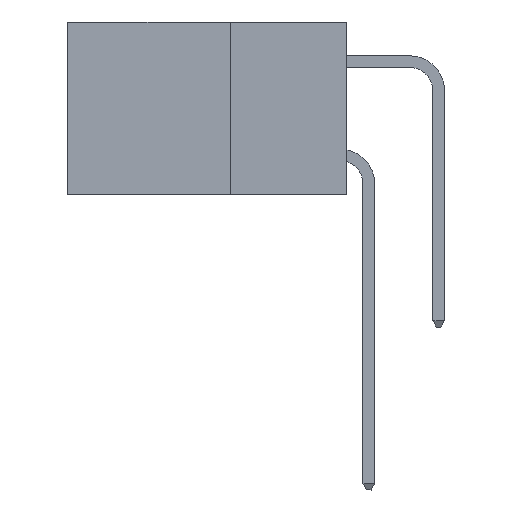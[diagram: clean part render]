
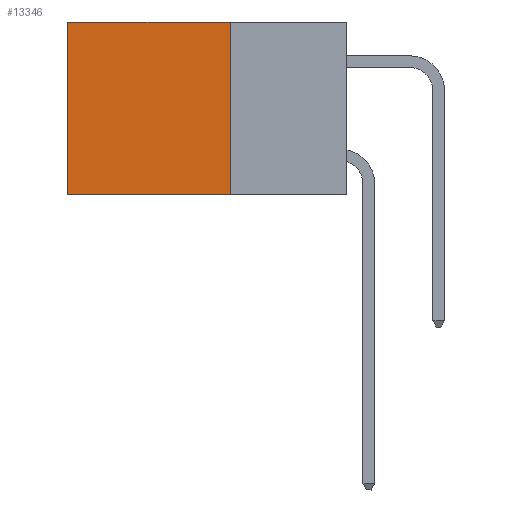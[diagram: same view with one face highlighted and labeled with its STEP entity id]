
A CAD part, left-side view. The second image highlights one B-rep face of the part: STEP entity #13346.
In plain terms, the highlighted planar face has unit normal (-1, 0, 0).
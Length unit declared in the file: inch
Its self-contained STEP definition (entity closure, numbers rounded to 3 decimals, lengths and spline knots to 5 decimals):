
#24 = LINE ( 'NONE', #17422, #7165 ) ;
#796 = DIRECTION ( 'NONE',  ( 0., 1., 0. ) ) ;
#1942 = DIRECTION ( 'NONE',  ( 0., 1., 0. ) ) ;
#2718 = LINE ( 'NONE', #18324, #11036 ) ;
#2976 = DIRECTION ( 'NONE',  ( 0., 0., -1. ) ) ;
#3465 = VECTOR ( 'NONE', #2976, 39.37008 ) ;
#4637 = CARTESIAN_POINT ( 'NONE',  ( 0.2875, 0.25, 0. ) ) ;
#5913 = AXIS2_PLACEMENT_3D ( 'NONE', #19322, #11659, #7561 ) ;
#7165 = VECTOR ( 'NONE', #1942, 39.37008 ) ;
#7546 = EDGE_CURVE ( 'NONE', #17994, #19937, #24, .T. ) ;
#7561 = DIRECTION ( 'NONE',  ( 0., 0., -1. ) ) ;
#7886 = CARTESIAN_POINT ( 'NONE',  ( 0.2875, 0.6, 0. ) ) ;
#10501 = CARTESIAN_POINT ( 'NONE',  ( 0.2875, 0.6, -0.37 ) ) ;
#11036 = VECTOR ( 'NONE', #796, 39.37008 ) ;
#11659 = DIRECTION ( 'NONE',  ( 1., 0., 0. ) ) ;
#12599 = EDGE_LOOP ( 'NONE', ( #22197, #15051, #13017, #24459 ) ) ;
#13017 = ORIENTED_EDGE ( 'NONE', *, *, #17005, .F. ) ;
#13346 = ADVANCED_FACE ( 'NONE', ( #22930 ), #25240, .F. ) ;
#14143 = LINE ( 'NONE', #7886, #21385 ) ;
#15051 = ORIENTED_EDGE ( 'NONE', *, *, #24342, .F. ) ;
#15618 = EDGE_CURVE ( 'NONE', #19937, #22128, #14143, .T. ) ;
#16440 = CARTESIAN_POINT ( 'NONE',  ( 0.2875, 0.25, 0. ) ) ;
#17005 = EDGE_CURVE ( 'NONE', #17994, #24749, #20509, .T. ) ;
#17422 = CARTESIAN_POINT ( 'NONE',  ( 0.2875, 0.25, 0. ) ) ;
#17994 = VERTEX_POINT ( 'NONE', #16440 ) ;
#18324 = CARTESIAN_POINT ( 'NONE',  ( 0.2875, 0.25, -0.37 ) ) ;
#19322 = CARTESIAN_POINT ( 'NONE',  ( 0.2875, 0.25, 0. ) ) ;
#19937 = VERTEX_POINT ( 'NONE', #24118 ) ;
#20509 = LINE ( 'NONE', #4637, #3465 ) ;
#20952 = CARTESIAN_POINT ( 'NONE',  ( 0.2875, 0.25, -0.37 ) ) ;
#21385 = VECTOR ( 'NONE', #21704, 39.37008 ) ;
#21704 = DIRECTION ( 'NONE',  ( 0., 0., -1. ) ) ;
#22128 = VERTEX_POINT ( 'NONE', #10501 ) ;
#22197 = ORIENTED_EDGE ( 'NONE', *, *, #15618, .T. ) ;
#22930 = FACE_OUTER_BOUND ( 'NONE', #12599, .T. ) ;
#24118 = CARTESIAN_POINT ( 'NONE',  ( 0.2875, 0.6, 0. ) ) ;
#24342 = EDGE_CURVE ( 'NONE', #24749, #22128, #2718, .T. ) ;
#24459 = ORIENTED_EDGE ( 'NONE', *, *, #7546, .T. ) ;
#24749 = VERTEX_POINT ( 'NONE', #20952 ) ;
#25240 = PLANE ( 'NONE',  #5913 ) ;
